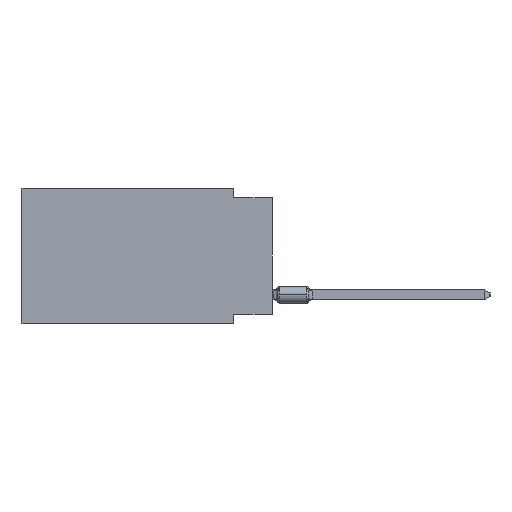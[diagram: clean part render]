
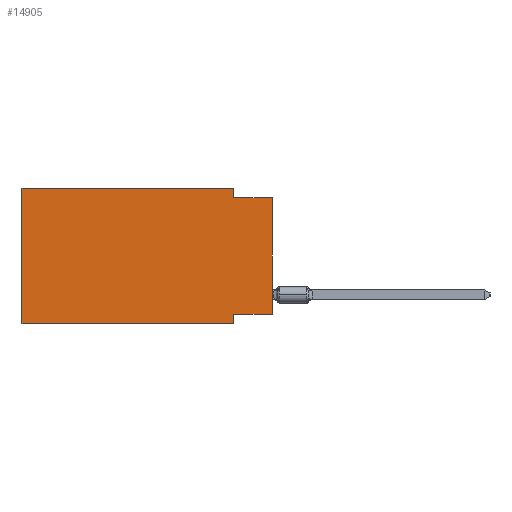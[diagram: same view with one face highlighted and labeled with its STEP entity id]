
A CAD part, left-side view. The second image highlights one B-rep face of the part: STEP entity #14905.
In plain terms, the highlighted planar face has unit normal (-1, 0, 0).
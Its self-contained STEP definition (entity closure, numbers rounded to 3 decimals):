
#890 = DIRECTION ( 'NONE',  ( 0., 0., -1. ) ) ;
#1498 = DIRECTION ( 'NONE',  ( 0., 1., 0. ) ) ;
#1685 = DIRECTION ( 'NONE',  ( 0., -1., 0. ) ) ;
#2434 = EDGE_CURVE ( 'NONE', #29482, #31221, #3788, .T. ) ;
#2996 = DIRECTION ( 'NONE',  ( 1., 0., 0. ) ) ;
#3788 = LINE ( 'NONE', #13972, #7036 ) ;
#4347 = CARTESIAN_POINT ( 'NONE',  ( 0., 16.383, -8.89 ) ) ;
#5394 = VECTOR ( 'NONE', #22135, 1000. ) ;
#7036 = VECTOR ( 'NONE', #1685, 1000. ) ;
#7453 = CARTESIAN_POINT ( 'NONE',  ( 0., 16.383, 0. ) ) ;
#7904 = VERTEX_POINT ( 'NONE', #26140 ) ;
#8556 = EDGE_CURVE ( 'NONE', #19165, #20641, #27382, .T. ) ;
#8969 = EDGE_CURVE ( 'NONE', #22867, #10123, #22481, .T. ) ;
#8999 = ORIENTED_EDGE ( 'NONE', *, *, #14058, .T. ) ;
#9890 = CARTESIAN_POINT ( 'NONE',  ( 0., 2.54, -8.89 ) ) ;
#9904 = CARTESIAN_POINT ( 'NONE',  ( 0., 0., 0. ) ) ;
#10123 = VERTEX_POINT ( 'NONE', #15208 ) ;
#10218 = DIRECTION ( 'NONE',  ( 0., 0., 1. ) ) ;
#12199 = ORIENTED_EDGE ( 'NONE', *, *, #8556, .F. ) ;
#12310 = EDGE_CURVE ( 'NONE', #7904, #16100, #20948, .T. ) ;
#12475 = EDGE_CURVE ( 'NONE', #16100, #31221, #24178, .T. ) ;
#12702 = FACE_OUTER_BOUND ( 'NONE', #29104, .T. ) ;
#12781 = DIRECTION ( 'NONE',  ( 0., -1., 0. ) ) ;
#12857 = VECTOR ( 'NONE', #28996, 1000. ) ;
#12978 = LINE ( 'NONE', #9904, #19412 ) ;
#13017 = CARTESIAN_POINT ( 'NONE',  ( 0., 16.383, 0. ) ) ;
#13202 = EDGE_CURVE ( 'NONE', #29482, #19165, #20022, .T. ) ;
#13320 = ORIENTED_EDGE ( 'NONE', *, *, #2434, .T. ) ;
#13753 = CARTESIAN_POINT ( 'NONE',  ( 0., 2.54, 0. ) ) ;
#13972 = CARTESIAN_POINT ( 'NONE',  ( 0., 16.383, -8.89 ) ) ;
#14058 = EDGE_CURVE ( 'NONE', #7904, #10123, #12978, .T. ) ;
#14905 = ADVANCED_FACE ( 'NONE', ( #12702 ), #20167, .F. ) ;
#15199 = AXIS2_PLACEMENT_3D ( 'NONE', #13017, #2996, #890 ) ;
#15208 = CARTESIAN_POINT ( 'NONE',  ( 0., 0., -0.635 ) ) ;
#16100 = VERTEX_POINT ( 'NONE', #18421 ) ;
#17068 = CARTESIAN_POINT ( 'NONE',  ( 0., 16.383, 0. ) ) ;
#18421 = CARTESIAN_POINT ( 'NONE',  ( 0., 2.54, -8.255 ) ) ;
#18776 = VECTOR ( 'NONE', #12781, 1000. ) ;
#18988 = CARTESIAN_POINT ( 'NONE',  ( 0., 0., -8.255 ) ) ;
#19165 = VERTEX_POINT ( 'NONE', #17068 ) ;
#19340 = ORIENTED_EDGE ( 'NONE', *, *, #13202, .F. ) ;
#19412 = VECTOR ( 'NONE', #10218, 1000. ) ;
#19712 = CARTESIAN_POINT ( 'NONE',  ( 0., 16.383, 0. ) ) ;
#20022 = LINE ( 'NONE', #19712, #5394 ) ;
#20167 = PLANE ( 'NONE',  #15199 ) ;
#20347 = VECTOR ( 'NONE', #31890, 1000. ) ;
#20641 = VERTEX_POINT ( 'NONE', #29391 ) ;
#20948 = LINE ( 'NONE', #18988, #22414 ) ;
#22135 = DIRECTION ( 'NONE',  ( 0., 0., 1. ) ) ;
#22414 = VECTOR ( 'NONE', #1498, 1000. ) ;
#22439 = CARTESIAN_POINT ( 'NONE',  ( 0., 2.54, -8.89 ) ) ;
#22481 = LINE ( 'NONE', #27507, #20347 ) ;
#22867 = VERTEX_POINT ( 'NONE', #31038 ) ;
#24178 = LINE ( 'NONE', #9890, #28128 ) ;
#26140 = CARTESIAN_POINT ( 'NONE',  ( 0., 0., -8.255 ) ) ;
#26295 = ORIENTED_EDGE ( 'NONE', *, *, #12310, .F. ) ;
#26673 = ORIENTED_EDGE ( 'NONE', *, *, #28764, .F. ) ;
#27382 = LINE ( 'NONE', #7453, #18776 ) ;
#27507 = CARTESIAN_POINT ( 'NONE',  ( 0., 0., -0.635 ) ) ;
#28128 = VECTOR ( 'NONE', #29668, 1000. ) ;
#28764 = EDGE_CURVE ( 'NONE', #20641, #22867, #31101, .T. ) ;
#28996 = DIRECTION ( 'NONE',  ( 0., 0., -1. ) ) ;
#29104 = EDGE_LOOP ( 'NONE', ( #8999, #29474, #26673, #12199, #19340, #13320, #31840, #26295 ) ) ;
#29391 = CARTESIAN_POINT ( 'NONE',  ( 0., 2.54, 0. ) ) ;
#29474 = ORIENTED_EDGE ( 'NONE', *, *, #8969, .F. ) ;
#29482 = VERTEX_POINT ( 'NONE', #4347 ) ;
#29668 = DIRECTION ( 'NONE',  ( 0., 0., -1. ) ) ;
#31038 = CARTESIAN_POINT ( 'NONE',  ( 0., 2.54, -0.635 ) ) ;
#31101 = LINE ( 'NONE', #13753, #12857 ) ;
#31221 = VERTEX_POINT ( 'NONE', #22439 ) ;
#31840 = ORIENTED_EDGE ( 'NONE', *, *, #12475, .F. ) ;
#31890 = DIRECTION ( 'NONE',  ( 0., -1., 0. ) ) ;
